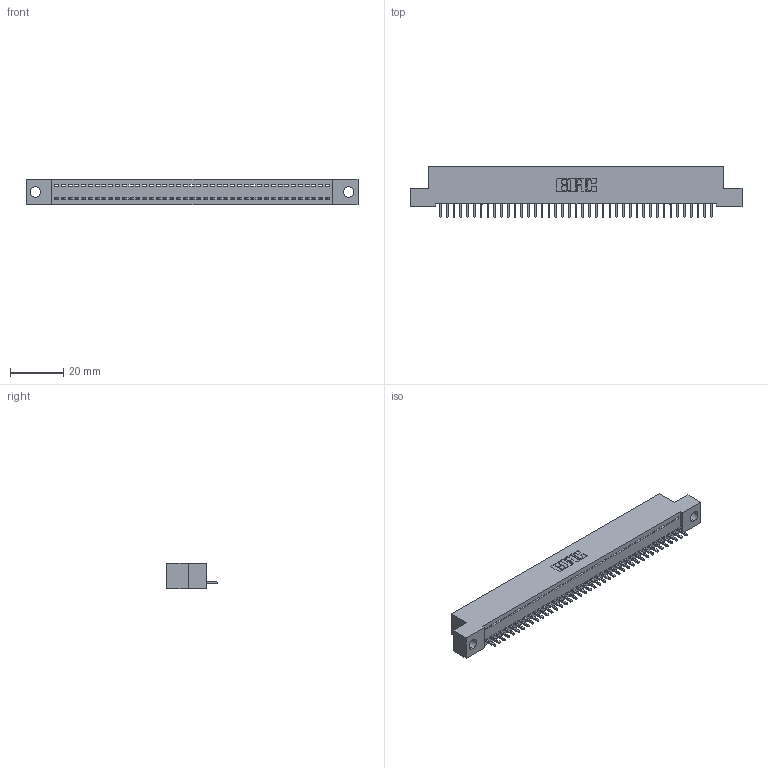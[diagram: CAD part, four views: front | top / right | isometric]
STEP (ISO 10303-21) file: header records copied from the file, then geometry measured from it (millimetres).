
FILE_DESCRIPTION (( 'STEP AP203' ), '1' );
FILE_NAME ('392-041-521-104.STEP', '2019-10-07T20:27:11', ( '' ), ( '' ), 'SwSTEP 2.0', 'SolidWorks 2016', '' );
FILE_SCHEMA (( 'CONFIG_CONTROL_DESIGN' ));
Length unit declared in the file: inch
Products named in the file (3): 342 Part_.156 TH; 345-292-001_345-293-121; 392-041-521-104
Assembly tree (42 placements, depth 2):
  392-041-521-104
    342 Part_.156 TH
    345-292-001_345-293-121  x41
Bounding box: 124.46 x 19.06 x 9.4 mm (x, y, z)
Volume: 10705.3 mm3; surface area: 15072.6 mm2
Topology: 42 solids, 42 shells, 2488 faces, 7515 edges, 4954 vertices
Faces by surface type: plane 1788, cylinder 700
Entity records: 25083 total; most frequent: CARTESIAN_POINT 4333, ORIENTED_EDGE 4310, DIRECTION 3657, EDGE_CURVE 2155, VECTOR 2027, LINE 2027, VERTEX_POINT 1434, AXIS2_PLACEMENT_3D 815
